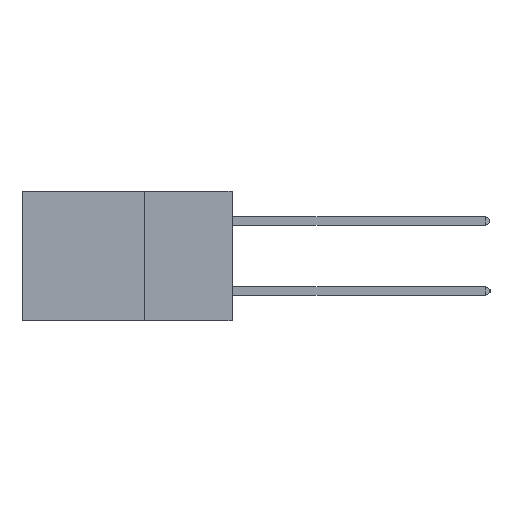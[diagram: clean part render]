
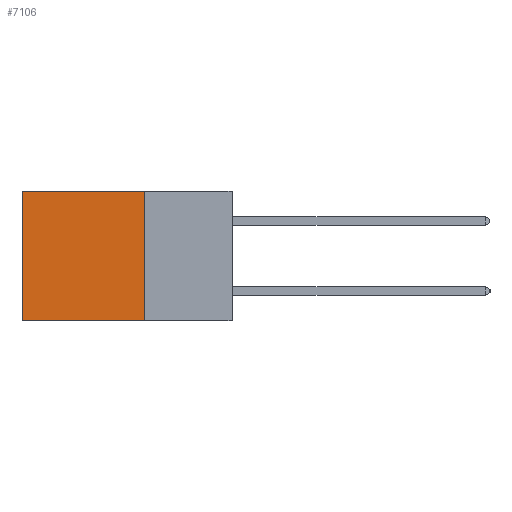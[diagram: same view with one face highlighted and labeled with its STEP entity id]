
A CAD part, left-side view. The second image highlights one B-rep face of the part: STEP entity #7106.
In plain terms, the highlighted planar face has unit normal (-1, 0, 0).
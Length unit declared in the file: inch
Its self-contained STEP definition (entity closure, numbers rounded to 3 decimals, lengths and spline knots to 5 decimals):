
#121 = VECTOR ( 'NONE', #23865, 39.37008 ) ;
#419 = ORIENTED_EDGE ( 'NONE', *, *, #23679, .F. ) ;
#856 = VERTEX_POINT ( 'NONE', #5820 ) ;
#1074 = CARTESIAN_POINT ( 'NONE',  ( 0.2875, 0.6, -0.37 ) ) ;
#3175 = PLANE ( 'NONE',  #11121 ) ;
#3253 = CARTESIAN_POINT ( 'NONE',  ( 0.2875, 0.25, 0. ) ) ;
#3624 = LINE ( 'NONE', #16809, #7980 ) ;
#5550 = EDGE_LOOP ( 'NONE', ( #10640, #14643, #419, #23981 ) ) ;
#5820 = CARTESIAN_POINT ( 'NONE',  ( 0.2875, 0.25, -0.37 ) ) ;
#7106 = ADVANCED_FACE ( 'NONE', ( #20650 ), #3175, .F. ) ;
#7389 = LINE ( 'NONE', #14750, #21896 ) ;
#7885 = DIRECTION ( 'NONE',  ( 0., 1., 0. ) ) ;
#7980 = VECTOR ( 'NONE', #14949, 39.37008 ) ;
#10485 = VERTEX_POINT ( 'NONE', #10822 ) ;
#10610 = DIRECTION ( 'NONE',  ( 0., 1., 0. ) ) ;
#10632 = CARTESIAN_POINT ( 'NONE',  ( 0.2875, 0.25, 0. ) ) ;
#10640 = ORIENTED_EDGE ( 'NONE', *, *, #14760, .T. ) ;
#10822 = CARTESIAN_POINT ( 'NONE',  ( 0.2875, 0.6, 0. ) ) ;
#11121 = AXIS2_PLACEMENT_3D ( 'NONE', #24333, #16546, #20439 ) ;
#11129 = VECTOR ( 'NONE', #10610, 39.37008 ) ;
#11300 = CARTESIAN_POINT ( 'NONE',  ( 0.2875, 0.25, 0. ) ) ;
#14643 = ORIENTED_EDGE ( 'NONE', *, *, #21825, .F. ) ;
#14750 = CARTESIAN_POINT ( 'NONE',  ( 0.2875, 0.25, -0.37 ) ) ;
#14760 = EDGE_CURVE ( 'NONE', #10485, #20484, #3624, .T. ) ;
#14949 = DIRECTION ( 'NONE',  ( 0., 0., -1. ) ) ;
#14973 = LINE ( 'NONE', #10632, #121 ) ;
#15007 = LINE ( 'NONE', #3253, #11129 ) ;
#16546 = DIRECTION ( 'NONE',  ( 1., 0., 0. ) ) ;
#16809 = CARTESIAN_POINT ( 'NONE',  ( 0.2875, 0.6, 0. ) ) ;
#18403 = EDGE_CURVE ( 'NONE', #20689, #10485, #15007, .T. ) ;
#20439 = DIRECTION ( 'NONE',  ( 0., 0., -1. ) ) ;
#20484 = VERTEX_POINT ( 'NONE', #1074 ) ;
#20650 = FACE_OUTER_BOUND ( 'NONE', #5550, .T. ) ;
#20689 = VERTEX_POINT ( 'NONE', #11300 ) ;
#21825 = EDGE_CURVE ( 'NONE', #856, #20484, #7389, .T. ) ;
#21896 = VECTOR ( 'NONE', #7885, 39.37008 ) ;
#23679 = EDGE_CURVE ( 'NONE', #20689, #856, #14973, .T. ) ;
#23865 = DIRECTION ( 'NONE',  ( 0., 0., -1. ) ) ;
#23981 = ORIENTED_EDGE ( 'NONE', *, *, #18403, .T. ) ;
#24333 = CARTESIAN_POINT ( 'NONE',  ( 0.2875, 0.25, 0. ) ) ;
